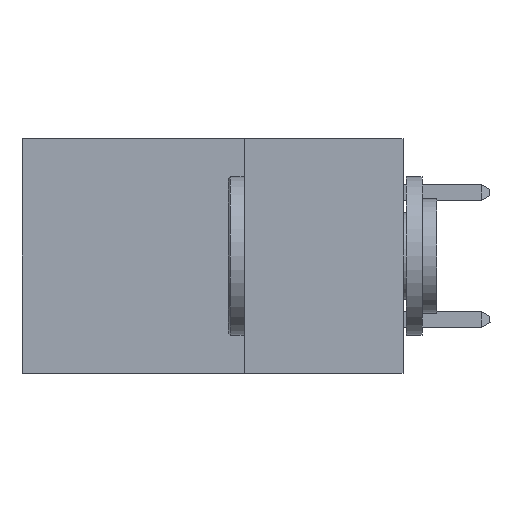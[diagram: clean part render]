
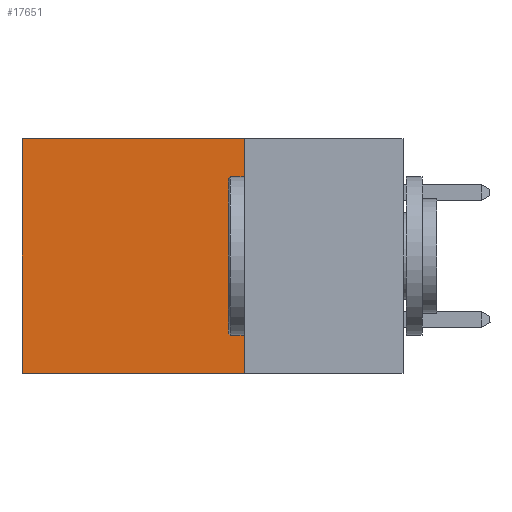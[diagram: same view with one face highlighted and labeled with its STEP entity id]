
A CAD part, left-side view. The second image highlights one B-rep face of the part: STEP entity #17651.
In plain terms, the highlighted planar face has unit normal (-1, 0, 0).
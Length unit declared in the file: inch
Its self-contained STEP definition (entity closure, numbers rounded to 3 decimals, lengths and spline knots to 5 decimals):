
#272 = DIRECTION ( 'NONE',  ( 0., 1., 0. ) ) ;
#676 = EDGE_LOOP ( 'NONE', ( #8484, #1877, #1670, #24009 ) ) ;
#1581 = EDGE_CURVE ( 'NONE', #4989, #22887, #19973, .T. ) ;
#1670 = ORIENTED_EDGE ( 'NONE', *, *, #24314, .F. ) ;
#1711 = EDGE_CURVE ( 'NONE', #25040, #4232, #25128, .T. ) ;
#1877 = ORIENTED_EDGE ( 'NONE', *, *, #1711, .F. ) ;
#3250 = VECTOR ( 'NONE', #14955, 39.37008 ) ;
#4232 = VERTEX_POINT ( 'NONE', #6012 ) ;
#4236 = CARTESIAN_POINT ( 'NONE',  ( 0.2875, 0.25, 0. ) ) ;
#4989 = VERTEX_POINT ( 'NONE', #16795 ) ;
#5886 = LINE ( 'NONE', #16139, #21795 ) ;
#6012 = CARTESIAN_POINT ( 'NONE',  ( 0.2875, 0.6, -0.37 ) ) ;
#6366 = PLANE ( 'NONE',  #22631 ) ;
#8484 = ORIENTED_EDGE ( 'NONE', *, *, #8605, .T. ) ;
#8605 = EDGE_CURVE ( 'NONE', #22887, #4232, #17439, .T. ) ;
#9355 = CARTESIAN_POINT ( 'NONE',  ( 0.2875, 0.6, 0. ) ) ;
#9391 = DIRECTION ( 'NONE',  ( 0., 0., -1. ) ) ;
#10299 = CARTESIAN_POINT ( 'NONE',  ( 0.2875, 0.25, -0.37 ) ) ;
#12376 = DIRECTION ( 'NONE',  ( 0., 1., 0. ) ) ;
#14955 = DIRECTION ( 'NONE',  ( 0., 0., -1. ) ) ;
#16139 = CARTESIAN_POINT ( 'NONE',  ( 0.2875, 0.25, 0. ) ) ;
#16795 = CARTESIAN_POINT ( 'NONE',  ( 0.2875, 0.25, 0. ) ) ;
#17439 = LINE ( 'NONE', #9355, #3250 ) ;
#17561 = VECTOR ( 'NONE', #272, 39.37008 ) ;
#17651 = ADVANCED_FACE ( 'NONE', ( #20337 ), #6366, .F. ) ;
#19643 = VECTOR ( 'NONE', #12376, 39.37008 ) ;
#19973 = LINE ( 'NONE', #21649, #19643 ) ;
#20337 = FACE_OUTER_BOUND ( 'NONE', #676, .T. ) ;
#21649 = CARTESIAN_POINT ( 'NONE',  ( 0.2875, 0.25, 0. ) ) ;
#21795 = VECTOR ( 'NONE', #9391, 39.37008 ) ;
#22072 = DIRECTION ( 'NONE',  ( 0., 0., -1. ) ) ;
#22631 = AXIS2_PLACEMENT_3D ( 'NONE', #4236, #26504, #22072 ) ;
#22887 = VERTEX_POINT ( 'NONE', #27521 ) ;
#24009 = ORIENTED_EDGE ( 'NONE', *, *, #1581, .T. ) ;
#24314 = EDGE_CURVE ( 'NONE', #4989, #25040, #5886, .T. ) ;
#25040 = VERTEX_POINT ( 'NONE', #10299 ) ;
#25128 = LINE ( 'NONE', #26685, #17561 ) ;
#26504 = DIRECTION ( 'NONE',  ( 1., 0., 0. ) ) ;
#26685 = CARTESIAN_POINT ( 'NONE',  ( 0.2875, 0.25, -0.37 ) ) ;
#27521 = CARTESIAN_POINT ( 'NONE',  ( 0.2875, 0.6, 0. ) ) ;
